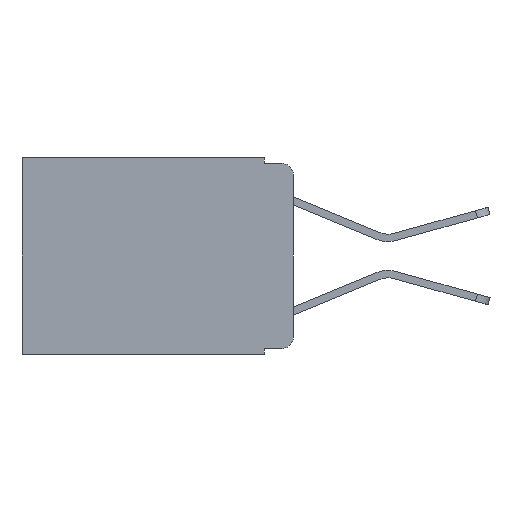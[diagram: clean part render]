
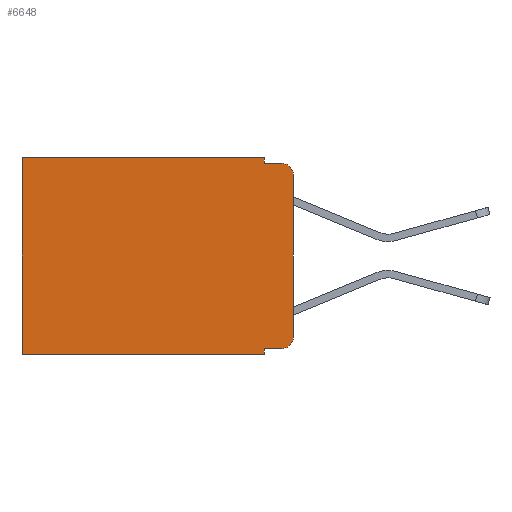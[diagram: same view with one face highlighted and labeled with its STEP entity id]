
A CAD part, left-side view. The second image highlights one B-rep face of the part: STEP entity #6648.
In plain terms, the highlighted planar face has unit normal (-1, 0, 0).
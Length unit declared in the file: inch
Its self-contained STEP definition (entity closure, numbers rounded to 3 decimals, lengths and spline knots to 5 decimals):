
#28 = DIRECTION ( 'NONE',  ( 1., 0., 0. ) ) ;
#757 = ORIENTED_EDGE ( 'NONE', *, *, #12802, .F. ) ;
#858 = CARTESIAN_POINT ( 'NONE',  ( 0.298, 0.02, -0.313 ) ) ;
#962 = FACE_OUTER_BOUND ( 'NONE', #4306, .T. ) ;
#965 = CARTESIAN_POINT ( 'NONE',  ( 0.298, 0.051, -0.01 ) ) ;
#1015 = ORIENTED_EDGE ( 'NONE', *, *, #3412, .T. ) ;
#1163 = VECTOR ( 'NONE', #13288, 39.37008 ) ;
#1183 = DIRECTION ( 'NONE',  ( 0., 0., -1. ) ) ;
#1577 = VERTEX_POINT ( 'NONE', #13085 ) ;
#1786 = DIRECTION ( 'NONE',  ( 0., 1., 0. ) ) ;
#1918 = CARTESIAN_POINT ( 'NONE',  ( 0.298, 0.473, 0. ) ) ;
#1946 = VERTEX_POINT ( 'NONE', #965 ) ;
#2095 = CARTESIAN_POINT ( 'NONE',  ( 0.298, 0.473, -0.343 ) ) ;
#2222 = DIRECTION ( 'NONE',  ( 0., 0., -1. ) ) ;
#2407 = VERTEX_POINT ( 'NONE', #2095 ) ;
#2642 = VECTOR ( 'NONE', #10186, 39.37008 ) ;
#2705 = CARTESIAN_POINT ( 'NONE',  ( 0.298, 0., -0.343 ) ) ;
#2758 = VERTEX_POINT ( 'NONE', #13840 ) ;
#2922 = CIRCLE ( 'NONE', #10002, 0.02 ) ;
#2975 = VECTOR ( 'NONE', #13685, 39.37008 ) ;
#3044 = EDGE_CURVE ( 'NONE', #2758, #5657, #5703, .T. ) ;
#3311 = PLANE ( 'NONE',  #5382 ) ;
#3352 = LINE ( 'NONE', #10235, #2642 ) ;
#3378 = ORIENTED_EDGE ( 'NONE', *, *, #5161, .F. ) ;
#3412 = EDGE_CURVE ( 'NONE', #1577, #2407, #11721, .T. ) ;
#3501 = VERTEX_POINT ( 'NONE', #6485 ) ;
#3623 = ORIENTED_EDGE ( 'NONE', *, *, #10521, .T. ) ;
#3826 = CARTESIAN_POINT ( 'NONE',  ( 0.298, 0.051, 0. ) ) ;
#4152 = CARTESIAN_POINT ( 'NONE',  ( 0.298, 0., 0. ) ) ;
#4306 = EDGE_LOOP ( 'NONE', ( #3378, #13502, #757, #6331, #3623, #1015, #13325, #9072, #6749, #13858 ) ) ;
#4404 = CARTESIAN_POINT ( 'NONE',  ( 0.298, 0., 0. ) ) ;
#4489 = VECTOR ( 'NONE', #12831, 39.37008 ) ;
#4773 = VERTEX_POINT ( 'NONE', #7583 ) ;
#5147 = LINE ( 'NONE', #6735, #1163 ) ;
#5161 = EDGE_CURVE ( 'NONE', #2758, #3501, #5147, .T. ) ;
#5382 = AXIS2_PLACEMENT_3D ( 'NONE', #4404, #28, #1183 ) ;
#5550 = DIRECTION ( 'NONE',  ( -1., 0., 0. ) ) ;
#5657 = VERTEX_POINT ( 'NONE', #7039 ) ;
#5703 = CIRCLE ( 'NONE', #5788, 0.02 ) ;
#5788 = AXIS2_PLACEMENT_3D ( 'NONE', #8815, #5550, #2222 ) ;
#5880 = LINE ( 'NONE', #2705, #2975 ) ;
#6233 = DIRECTION ( 'NONE',  ( -1., 0., 0. ) ) ;
#6281 = DIRECTION ( 'NONE',  ( 0., 0., -1. ) ) ;
#6297 = EDGE_CURVE ( 'NONE', #4773, #10436, #13839, .T. ) ;
#6331 = ORIENTED_EDGE ( 'NONE', *, *, #10799, .F. ) ;
#6485 = CARTESIAN_POINT ( 'NONE',  ( 0.298, 0., -0.313 ) ) ;
#6648 = ADVANCED_FACE ( 'NONE', ( #962 ), #3311, .F. ) ;
#6735 = CARTESIAN_POINT ( 'NONE',  ( 0.298, 0., 0. ) ) ;
#6749 = ORIENTED_EDGE ( 'NONE', *, *, #8791, .T. ) ;
#7039 = CARTESIAN_POINT ( 'NONE',  ( 0.298, 0.02, -0.01 ) ) ;
#7160 = VECTOR ( 'NONE', #7756, 39.37008 ) ;
#7178 = VECTOR ( 'NONE', #1786, 39.37008 ) ;
#7218 = CARTESIAN_POINT ( 'NONE',  ( 0.298, 0.051, -0.343 ) ) ;
#7583 = CARTESIAN_POINT ( 'NONE',  ( 0.298, 0.051, -0.333 ) ) ;
#7756 = DIRECTION ( 'NONE',  ( 0., 0., -1. ) ) ;
#7963 = EDGE_CURVE ( 'NONE', #10436, #2407, #5880, .T. ) ;
#8791 = EDGE_CURVE ( 'NONE', #4773, #13896, #12044, .T. ) ;
#8815 = CARTESIAN_POINT ( 'NONE',  ( 0.298, 0.02, -0.03 ) ) ;
#9072 = ORIENTED_EDGE ( 'NONE', *, *, #6297, .F. ) ;
#9451 = VERTEX_POINT ( 'NONE', #3826 ) ;
#9820 = CARTESIAN_POINT ( 'NONE',  ( 0.298, 0.051, 0. ) ) ;
#10002 = AXIS2_PLACEMENT_3D ( 'NONE', #858, #6233, #10817 ) ;
#10022 = CARTESIAN_POINT ( 'NONE',  ( 0.298, 0.02, -0.333 ) ) ;
#10147 = EDGE_CURVE ( 'NONE', #13896, #3501, #2922, .T. ) ;
#10186 = DIRECTION ( 'NONE',  ( 0., -1., 0. ) ) ;
#10235 = CARTESIAN_POINT ( 'NONE',  ( 0.298, 0.051, -0.01 ) ) ;
#10432 = LINE ( 'NONE', #9820, #7160 ) ;
#10436 = VERTEX_POINT ( 'NONE', #7218 ) ;
#10493 = CARTESIAN_POINT ( 'NONE',  ( 0.298, 0.051, -0.333 ) ) ;
#10521 = EDGE_CURVE ( 'NONE', #9451, #1577, #13878, .T. ) ;
#10799 = EDGE_CURVE ( 'NONE', #9451, #1946, #10432, .T. ) ;
#10817 = DIRECTION ( 'NONE',  ( 0., 0., -1. ) ) ;
#11462 = VECTOR ( 'NONE', #6281, 39.37008 ) ;
#11721 = LINE ( 'NONE', #1918, #4489 ) ;
#11764 = CARTESIAN_POINT ( 'NONE',  ( 0.298, 0.051, 0. ) ) ;
#12044 = LINE ( 'NONE', #10493, #12380 ) ;
#12380 = VECTOR ( 'NONE', #12757, 39.37008 ) ;
#12757 = DIRECTION ( 'NONE',  ( 0., -1., 0. ) ) ;
#12802 = EDGE_CURVE ( 'NONE', #1946, #5657, #3352, .T. ) ;
#12831 = DIRECTION ( 'NONE',  ( 0., 0., -1. ) ) ;
#13085 = CARTESIAN_POINT ( 'NONE',  ( 0.298, 0.473, 0. ) ) ;
#13288 = DIRECTION ( 'NONE',  ( 0., 0., -1. ) ) ;
#13325 = ORIENTED_EDGE ( 'NONE', *, *, #7963, .F. ) ;
#13502 = ORIENTED_EDGE ( 'NONE', *, *, #3044, .T. ) ;
#13685 = DIRECTION ( 'NONE',  ( 0., 1., 0. ) ) ;
#13839 = LINE ( 'NONE', #11764, #11462 ) ;
#13840 = CARTESIAN_POINT ( 'NONE',  ( 0.298, 0., -0.03 ) ) ;
#13858 = ORIENTED_EDGE ( 'NONE', *, *, #10147, .T. ) ;
#13878 = LINE ( 'NONE', #4152, #7178 ) ;
#13896 = VERTEX_POINT ( 'NONE', #10022 ) ;
